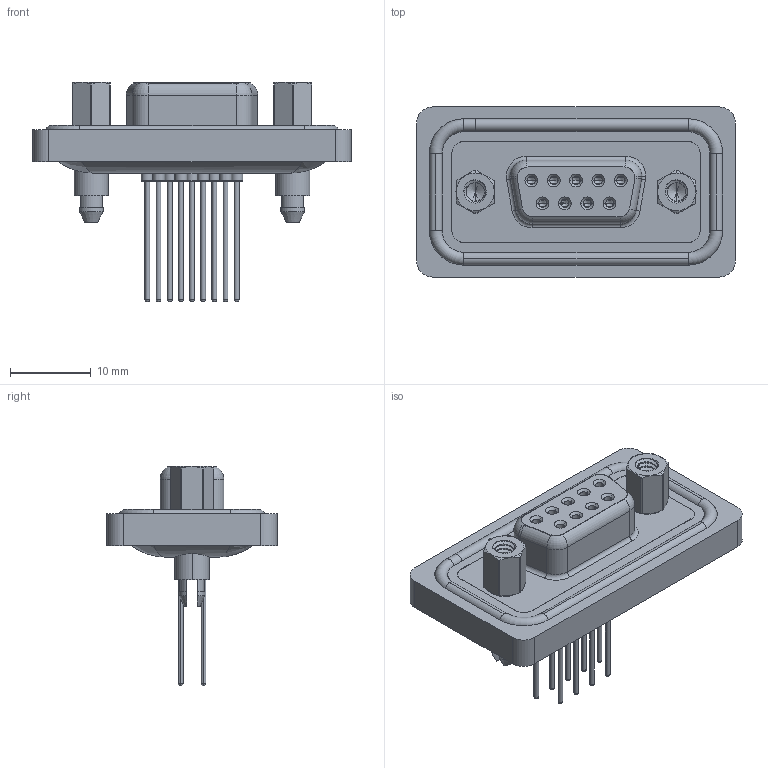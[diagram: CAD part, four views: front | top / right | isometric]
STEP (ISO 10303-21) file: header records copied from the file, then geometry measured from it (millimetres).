
FILE_DESCRIPTION (( 'STEP AP203' ), '1' );
FILE_NAME ('628-W09-321-013.STEP', '2020-09-11T23:18:14', ( '' ), ( '' ), 'SwSTEP 2.0', 'SolidWorks 2020', '' );
FILE_SCHEMA (( 'CONFIG_CONTROL_DESIGN' ));
Length unit declared in the file: millimetre
Products named in the file (8): 628-W09-321-013; 628W Housing_09 Contacts; 628W Contact Row 2_21; 628W Contact Row 1_21; 628W 4-40 Hex Standoff; 628W 4-40 Threaded Boardlock; 628W Shell Front_09 Contacts; 628W Waterproof Housing_09 Contacts BL
Assembly tree (16 placements, depth 2):
  628-W09-321-013
    628W Housing_09 Contacts
    628W Shell Front_09 Contacts
    628W Contact Row 1_21  x5
    628W Contact Row 2_21  x4
    628W 4-40 Threaded Boardlock  x2
    628W Waterproof Housing_09 Contacts BL
    628W 4-40 Hex Standoff  x2
Bounding box: 39.51 x 21.1 x 27.2 mm (x, y, z)
Volume: 4521.7 mm3; surface area: 7709.3 mm2
Topology: 17 solids, 17 shells, 982 faces, 2408 edges, 1507 vertices
Faces by surface type: cylinder 437, plane 250, torus 176, cone 97, bspline 22
Entity records: 22566 total; most frequent: CARTESIAN_POINT 7950, DIRECTION 2961, ORIENTED_EDGE 2778, EDGE_CURVE 1389, AXIS2_PLACEMENT_3D 1217, VERTEX_POINT 886, EDGE_LOOP 663, CIRCLE 644
